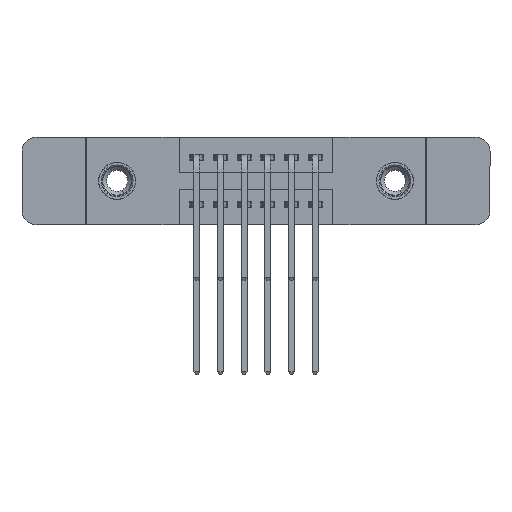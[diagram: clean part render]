
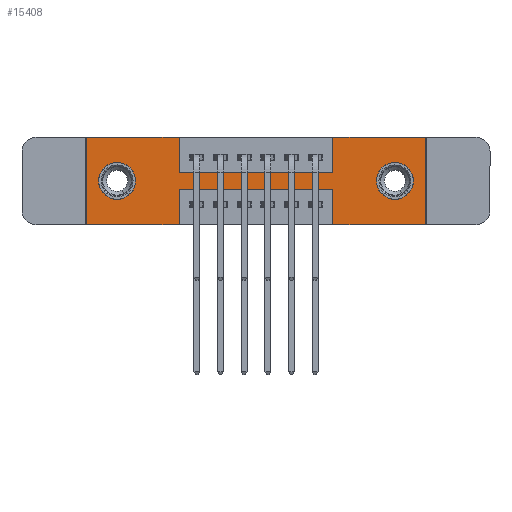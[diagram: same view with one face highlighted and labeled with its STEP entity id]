
A CAD part, front view. The second image highlights one B-rep face of the part: STEP entity #15408.
In plain terms, the highlighted planar face has unit normal (0, -1, 0).
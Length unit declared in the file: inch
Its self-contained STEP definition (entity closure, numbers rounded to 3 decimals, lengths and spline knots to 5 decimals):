
#114 = CARTESIAN_POINT ( 'NONE',  ( 1.435, 0., 0. ) ) ;
#259 = EDGE_CURVE ( 'NONE', #1585, #7829, #1854, .T. ) ;
#291 = LINE ( 'NONE', #777, #3475 ) ;
#348 = ORIENTED_EDGE ( 'NONE', *, *, #15902, .F. ) ;
#363 = LINE ( 'NONE', #3886, #5718 ) ;
#367 = VERTEX_POINT ( 'NONE', #6307 ) ;
#777 = CARTESIAN_POINT ( 'NONE',  ( 0., 0., 0. ) ) ;
#994 = EDGE_LOOP ( 'NONE', ( #13976, #13699 ) ) ;
#1015 = CIRCLE ( 'NONE', #15312, 0.078 ) ;
#1147 = DIRECTION ( 'NONE',  ( 0., 0., -1. ) ) ;
#1257 = CARTESIAN_POINT ( 'NONE',  ( 0., 0., -0.37 ) ) ;
#1573 = DIRECTION ( 'NONE',  ( -1., 0., 0. ) ) ;
#1585 = VERTEX_POINT ( 'NONE', #5799 ) ;
#1780 = DIRECTION ( 'NONE',  ( 0., 0., 1. ) ) ;
#1854 = LINE ( 'NONE', #9672, #7763 ) ;
#2027 = DIRECTION ( 'NONE',  ( -1., 0., 0. ) ) ;
#2039 = ORIENTED_EDGE ( 'NONE', *, *, #14852, .F. ) ;
#2194 = VECTOR ( 'NONE', #2027, 39.37008 ) ;
#2210 = CARTESIAN_POINT ( 'NONE',  ( 0.13, 0., -0.263 ) ) ;
#2263 = CARTESIAN_POINT ( 'NONE',  ( 1.0425, 0., 0. ) ) ;
#2393 = CARTESIAN_POINT ( 'NONE',  ( 1.0425, 0., -0.15 ) ) ;
#2451 = DIRECTION ( 'NONE',  ( 1., 0., 0. ) ) ;
#2603 = FACE_BOUND ( 'NONE', #11293, .T. ) ;
#2619 = DIRECTION ( 'NONE',  ( 0., 0., 1. ) ) ;
#2816 = CARTESIAN_POINT ( 'NONE',  ( 0.3925, 0., -0.37 ) ) ;
#2876 = EDGE_CURVE ( 'NONE', #11569, #14887, #16048, .T. ) ;
#3028 = DIRECTION ( 'NONE',  ( 0., 1., 0. ) ) ;
#3074 = PLANE ( 'NONE',  #8080 ) ;
#3167 = EDGE_CURVE ( 'NONE', #367, #11387, #6509, .T. ) ;
#3228 = AXIS2_PLACEMENT_3D ( 'NONE', #8164, #4188, #14314 ) ;
#3268 = VERTEX_POINT ( 'NONE', #11865 ) ;
#3362 = CARTESIAN_POINT ( 'NONE',  ( 0., 0., -0.37 ) ) ;
#3397 = FACE_BOUND ( 'NONE', #994, .T. ) ;
#3475 = VECTOR ( 'NONE', #2451, 39.37008 ) ;
#3481 = VERTEX_POINT ( 'NONE', #5886 ) ;
#3697 = EDGE_CURVE ( 'NONE', #14794, #15736, #363, .T. ) ;
#3758 = CARTESIAN_POINT ( 'NONE',  ( 1.435, 0., 0. ) ) ;
#3886 = CARTESIAN_POINT ( 'NONE',  ( 1.0425, 0., -0.37 ) ) ;
#3902 = DIRECTION ( 'NONE',  ( 1., 0., 0. ) ) ;
#3987 = ORIENTED_EDGE ( 'NONE', *, *, #3167, .T. ) ;
#4188 = DIRECTION ( 'NONE',  ( 0., 1., 0. ) ) ;
#4600 = DIRECTION ( 'NONE',  ( 0., 0., -1. ) ) ;
#4807 = ORIENTED_EDGE ( 'NONE', *, *, #11734, .F. ) ;
#4982 = DIRECTION ( 'NONE',  ( 0., 0., -1. ) ) ;
#5023 = ORIENTED_EDGE ( 'NONE', *, *, #14906, .F. ) ;
#5074 = LINE ( 'NONE', #1257, #8836 ) ;
#5171 = VERTEX_POINT ( 'NONE', #114 ) ;
#5242 = CARTESIAN_POINT ( 'NONE',  ( 0., 0., 0. ) ) ;
#5370 = LINE ( 'NONE', #3362, #2194 ) ;
#5696 = DIRECTION ( 'NONE',  ( 0., 0., -1. ) ) ;
#5718 = VECTOR ( 'NONE', #6373, 39.37008 ) ;
#5754 = ORIENTED_EDGE ( 'NONE', *, *, #2876, .F. ) ;
#5789 = DIRECTION ( 'NONE',  ( 0., 1., 0. ) ) ;
#5799 = CARTESIAN_POINT ( 'NONE',  ( 0., 0., -0.37 ) ) ;
#5854 = VECTOR ( 'NONE', #1147, 39.37008 ) ;
#5886 = CARTESIAN_POINT ( 'NONE',  ( 0.3925, 0., -0.22 ) ) ;
#6029 = AXIS2_PLACEMENT_3D ( 'NONE', #13974, #16328, #4982 ) ;
#6087 = CARTESIAN_POINT ( 'NONE',  ( 1.0425, 0., 0. ) ) ;
#6159 = VECTOR ( 'NONE', #6659, 39.37008 ) ;
#6170 = ORIENTED_EDGE ( 'NONE', *, *, #15630, .F. ) ;
#6307 = CARTESIAN_POINT ( 'NONE',  ( 1.305, 0., -0.263 ) ) ;
#6373 = DIRECTION ( 'NONE',  ( 0., 0., 1. ) ) ;
#6445 = EDGE_CURVE ( 'NONE', #7829, #11569, #291, .T. ) ;
#6509 = CIRCLE ( 'NONE', #3228, 0.078 ) ;
#6659 = DIRECTION ( 'NONE',  ( 0., 0., -1. ) ) ;
#6852 = ORIENTED_EDGE ( 'NONE', *, *, #12506, .F. ) ;
#6860 = VERTEX_POINT ( 'NONE', #2210 ) ;
#6888 = VERTEX_POINT ( 'NONE', #2263 ) ;
#6979 = CARTESIAN_POINT ( 'NONE',  ( 0.3925, 0., 0. ) ) ;
#6988 = DIRECTION ( 'NONE',  ( 0., 0., 1. ) ) ;
#7040 = DIRECTION ( 'NONE',  ( 0., 0., 1. ) ) ;
#7221 = CIRCLE ( 'NONE', #6029, 0.078 ) ;
#7495 = ORIENTED_EDGE ( 'NONE', *, *, #6445, .F. ) ;
#7537 = CARTESIAN_POINT ( 'NONE',  ( 1.0425, 0., -0.37 ) ) ;
#7640 = VERTEX_POINT ( 'NONE', #8628 ) ;
#7666 = DIRECTION ( 'NONE',  ( -1., 0., 0. ) ) ;
#7683 = VERTEX_POINT ( 'NONE', #2393 ) ;
#7763 = VECTOR ( 'NONE', #6988, 39.37008 ) ;
#7829 = VERTEX_POINT ( 'NONE', #13885 ) ;
#8080 = AXIS2_PLACEMENT_3D ( 'NONE', #10710, #10758, #5696 ) ;
#8132 = EDGE_CURVE ( 'NONE', #13632, #6860, #1015, .T. ) ;
#8159 = CARTESIAN_POINT ( 'NONE',  ( 0.13, 0., -0.185 ) ) ;
#8164 = CARTESIAN_POINT ( 'NONE',  ( 1.305, 0., -0.185 ) ) ;
#8178 = ORIENTED_EDGE ( 'NONE', *, *, #259, .F. ) ;
#8628 = CARTESIAN_POINT ( 'NONE',  ( 0.3925, 0., -0.37 ) ) ;
#8836 = VECTOR ( 'NONE', #7666, 39.37008 ) ;
#9117 = CARTESIAN_POINT ( 'NONE',  ( 1.0425, 0., -0.22 ) ) ;
#9218 = CARTESIAN_POINT ( 'NONE',  ( 0.3925, 0., -0.22 ) ) ;
#9239 = DIRECTION ( 'NONE',  ( 1., 0., 0. ) ) ;
#9405 = CARTESIAN_POINT ( 'NONE',  ( 0.13, 0., -0.185 ) ) ;
#9672 = CARTESIAN_POINT ( 'NONE',  ( 0., 0., 0. ) ) ;
#9679 = ORIENTED_EDGE ( 'NONE', *, *, #15296, .F. ) ;
#10271 = AXIS2_PLACEMENT_3D ( 'NONE', #8159, #5789, #7040 ) ;
#10349 = CARTESIAN_POINT ( 'NONE',  ( 0.3925, 0., -0.15 ) ) ;
#10496 = VECTOR ( 'NONE', #9239, 39.37008 ) ;
#10710 = CARTESIAN_POINT ( 'NONE',  ( 0., 0., -0.37 ) ) ;
#10716 = VECTOR ( 'NONE', #1573, 39.37008 ) ;
#10727 = EDGE_LOOP ( 'NONE', ( #5023, #2039, #13713, #15298, #6852, #6170, #4807, #9679, #5754, #7495, #8178, #348 ) ) ;
#10758 = DIRECTION ( 'NONE',  ( 0., -1., 0. ) ) ;
#11106 = LINE ( 'NONE', #9218, #10716 ) ;
#11272 = FACE_OUTER_BOUND ( 'NONE', #10727, .T. ) ;
#11293 = EDGE_LOOP ( 'NONE', ( #14562, #3987 ) ) ;
#11387 = VERTEX_POINT ( 'NONE', #11510 ) ;
#11510 = CARTESIAN_POINT ( 'NONE',  ( 1.305, 0., -0.107 ) ) ;
#11569 = VERTEX_POINT ( 'NONE', #13284 ) ;
#11611 = CARTESIAN_POINT ( 'NONE',  ( 0.13, 0., -0.107 ) ) ;
#11734 = EDGE_CURVE ( 'NONE', #7683, #6888, #12209, .T. ) ;
#11865 = CARTESIAN_POINT ( 'NONE',  ( 1.435, 0., -0.37 ) ) ;
#11870 = CIRCLE ( 'NONE', #10271, 0.078 ) ;
#12209 = LINE ( 'NONE', #6087, #15970 ) ;
#12443 = EDGE_CURVE ( 'NONE', #11387, #367, #7221, .T. ) ;
#12465 = EDGE_CURVE ( 'NONE', #3268, #14794, #5074, .T. ) ;
#12506 = EDGE_CURVE ( 'NONE', #5171, #3268, #15157, .T. ) ;
#12641 = VECTOR ( 'NONE', #4600, 39.37008 ) ;
#12861 = VECTOR ( 'NONE', #3902, 39.37008 ) ;
#13284 = CARTESIAN_POINT ( 'NONE',  ( 0.3925, 0., 0. ) ) ;
#13632 = VERTEX_POINT ( 'NONE', #11611 ) ;
#13699 = ORIENTED_EDGE ( 'NONE', *, *, #15923, .T. ) ;
#13713 = ORIENTED_EDGE ( 'NONE', *, *, #3697, .F. ) ;
#13866 = LINE ( 'NONE', #14274, #10496 ) ;
#13885 = CARTESIAN_POINT ( 'NONE',  ( 0., 0., 0. ) ) ;
#13974 = CARTESIAN_POINT ( 'NONE',  ( 1.305, 0., -0.185 ) ) ;
#13976 = ORIENTED_EDGE ( 'NONE', *, *, #8132, .T. ) ;
#14274 = CARTESIAN_POINT ( 'NONE',  ( 0.3925, 0., -0.15 ) ) ;
#14314 = DIRECTION ( 'NONE',  ( 0., 0., -1. ) ) ;
#14486 = LINE ( 'NONE', #2816, #6159 ) ;
#14562 = ORIENTED_EDGE ( 'NONE', *, *, #12443, .T. ) ;
#14794 = VERTEX_POINT ( 'NONE', #7537 ) ;
#14852 = EDGE_CURVE ( 'NONE', #15736, #3481, #11106, .T. ) ;
#14887 = VERTEX_POINT ( 'NONE', #10349 ) ;
#14906 = EDGE_CURVE ( 'NONE', #3481, #7640, #14486, .T. ) ;
#15157 = LINE ( 'NONE', #3758, #5854 ) ;
#15296 = EDGE_CURVE ( 'NONE', #14887, #7683, #13866, .T. ) ;
#15298 = ORIENTED_EDGE ( 'NONE', *, *, #12465, .F. ) ;
#15312 = AXIS2_PLACEMENT_3D ( 'NONE', #9405, #3028, #1780 ) ;
#15408 = ADVANCED_FACE ( 'NONE', ( #2603, #3397, #11272 ), #3074, .T. ) ;
#15630 = EDGE_CURVE ( 'NONE', #6888, #5171, #16258, .T. ) ;
#15736 = VERTEX_POINT ( 'NONE', #9117 ) ;
#15902 = EDGE_CURVE ( 'NONE', #7640, #1585, #5370, .T. ) ;
#15923 = EDGE_CURVE ( 'NONE', #6860, #13632, #11870, .T. ) ;
#15970 = VECTOR ( 'NONE', #2619, 39.37008 ) ;
#16048 = LINE ( 'NONE', #6979, #12641 ) ;
#16258 = LINE ( 'NONE', #5242, #12861 ) ;
#16328 = DIRECTION ( 'NONE',  ( 0., 1., 0. ) ) ;
